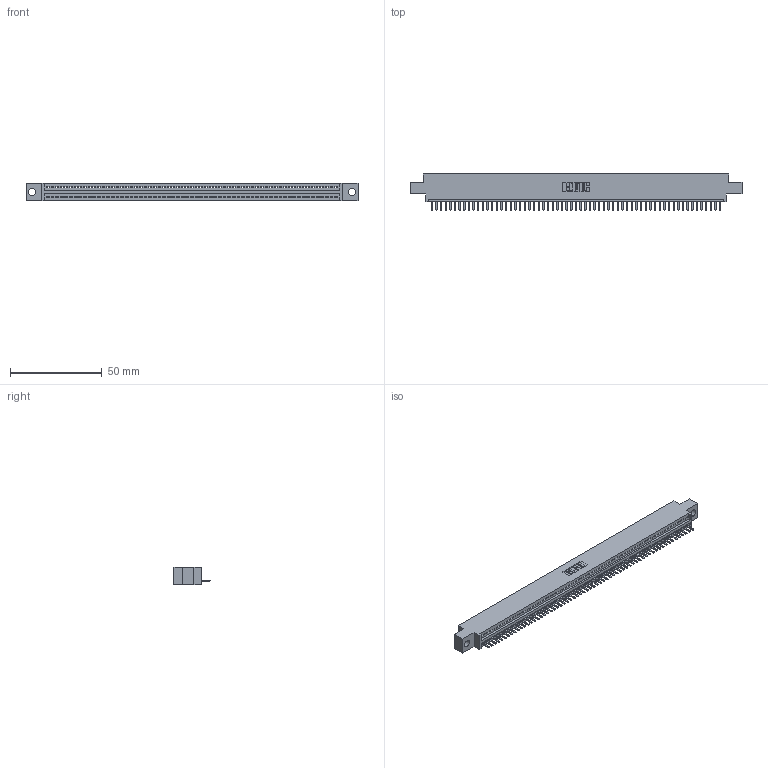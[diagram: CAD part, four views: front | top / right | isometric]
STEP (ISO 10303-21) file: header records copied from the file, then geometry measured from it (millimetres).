
FILE_DESCRIPTION (( 'STEP AP203' ), '1' );
FILE_NAME ('395-063-520-604.STEP', '2019-10-24T20:25:26', ( '' ), ( '' ), 'SwSTEP 2.0', 'SolidWorks 2016', '' );
FILE_SCHEMA (( 'CONFIG_CONTROL_DESIGN' ));
Length unit declared in the file: inch
Products named in the file (3): 345 Part_0.170 Offset - 0.156 Dia-TH; 395-063-520-604; 345-292-001_345-293-120
Assembly tree (64 placements, depth 2):
  395-063-520-604
    345 Part_0.170 Offset - 0.156 Dia-TH
    345-292-001_345-293-120  x63
Bounding box: 181.23 x 19.68 x 9.4 mm (x, y, z)
Volume: 17002.9 mm3; surface area: 22223.1 mm2
Topology: 64 solids, 64 shells, 4036 faces, 11945 edges, 7794 vertices
Faces by surface type: plane 2730, cylinder 1306
Entity records: 44837 total; most frequent: CARTESIAN_POINT 7785, ORIENTED_EDGE 7770, DIRECTION 6755, EDGE_CURVE 3885, VECTOR 3497, LINE 3497, VERTEX_POINT 2586, AXIS2_PLACEMENT_3D 1629
